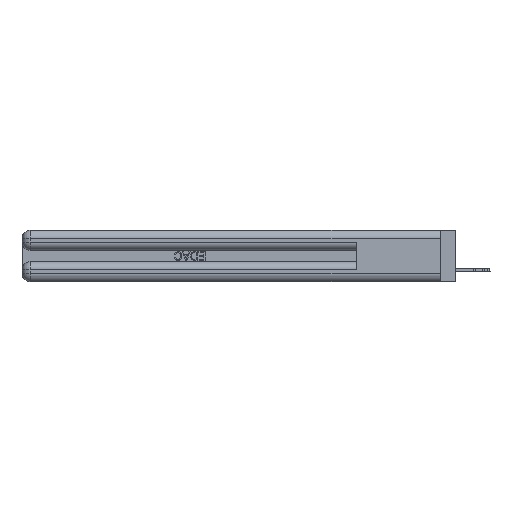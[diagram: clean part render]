
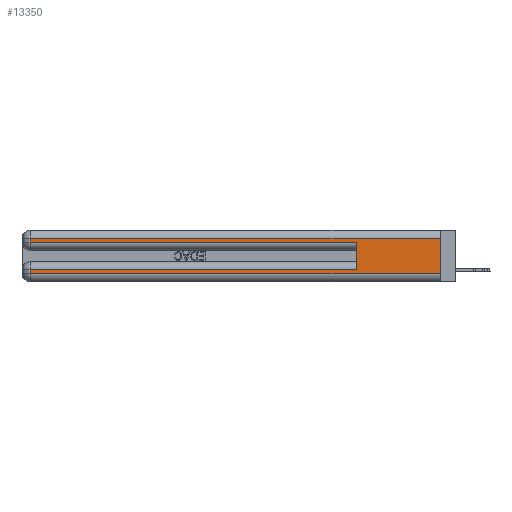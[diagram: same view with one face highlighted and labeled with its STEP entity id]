
A CAD part, left-side view. The second image highlights one B-rep face of the part: STEP entity #13350.
In plain terms, the highlighted planar face has unit normal (-1, 0, 0).
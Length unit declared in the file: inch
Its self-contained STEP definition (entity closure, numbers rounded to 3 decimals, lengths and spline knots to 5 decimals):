
#110 = DIRECTION ( 'NONE',  ( 0., 0., -1. ) ) ;
#806 = VERTEX_POINT ( 'NONE', #2833 ) ;
#1689 = VECTOR ( 'NONE', #25613, 39.37008 ) ;
#2033 = EDGE_CURVE ( 'NONE', #21175, #6465, #29939, .T. ) ;
#2107 = EDGE_CURVE ( 'NONE', #31301, #806, #5621, .T. ) ;
#2484 = FACE_OUTER_BOUND ( 'NONE', #23360, .T. ) ;
#2603 = DIRECTION ( 'NONE',  ( 0., 0., -1. ) ) ;
#2833 = CARTESIAN_POINT ( 'NONE',  ( 0., 2.94, 0.285 ) ) ;
#2837 = ORIENTED_EDGE ( 'NONE', *, *, #35792, .T. ) ;
#3821 = CARTESIAN_POINT ( 'NONE',  ( 0., 0., 0.085 ) ) ;
#3968 = DIRECTION ( 'NONE',  ( 0., 1., 0. ) ) ;
#4690 = ORIENTED_EDGE ( 'NONE', *, *, #9439, .F. ) ;
#5583 = AXIS2_PLACEMENT_3D ( 'NONE', #5845, #15861, #2603 ) ;
#5621 = LINE ( 'NONE', #41473, #11969 ) ;
#5845 = CARTESIAN_POINT ( 'NONE',  ( 0., 0., 0.37 ) ) ;
#6465 = VERTEX_POINT ( 'NONE', #33110 ) ;
#7440 = LINE ( 'NONE', #3821, #31172 ) ;
#9402 = CARTESIAN_POINT ( 'NONE',  ( 0., 2.94, 0.085 ) ) ;
#9439 = EDGE_CURVE ( 'NONE', #25438, #43082, #18098, .T. ) ;
#9541 = PLANE ( 'NONE',  #5583 ) ;
#10227 = VECTOR ( 'NONE', #19446, 39.37008 ) ;
#10429 = CARTESIAN_POINT ( 'NONE',  ( 0., 2.94, 0.31 ) ) ;
#11605 = CARTESIAN_POINT ( 'NONE',  ( 0., 2.94, 0.06 ) ) ;
#11969 = VECTOR ( 'NONE', #35269, 39.37008 ) ;
#12054 = CARTESIAN_POINT ( 'NONE',  ( 0., 0., 0.31 ) ) ;
#13350 = ADVANCED_FACE ( 'NONE', ( #2484 ), #9541, .F. ) ;
#14698 = EDGE_CURVE ( 'NONE', #25438, #38427, #7440, .T. ) ;
#15668 = CARTESIAN_POINT ( 'NONE',  ( 0., 0., 0.285 ) ) ;
#15861 = DIRECTION ( 'NONE',  ( 1., 0., 0. ) ) ;
#16443 = LINE ( 'NONE', #21924, #1689 ) ;
#16567 = CARTESIAN_POINT ( 'NONE',  ( 0., 0., 0.37 ) ) ;
#16701 = VECTOR ( 'NONE', #39273, 39.37008 ) ;
#17073 = EDGE_CURVE ( 'NONE', #38427, #19320, #24148, .T. ) ;
#17250 = CARTESIAN_POINT ( 'NONE',  ( 0., 0.6, 0.085 ) ) ;
#17826 = ORIENTED_EDGE ( 'NONE', *, *, #21265, .T. ) ;
#18098 = LINE ( 'NONE', #42594, #10227 ) ;
#19320 = VERTEX_POINT ( 'NONE', #11605 ) ;
#19446 = DIRECTION ( 'NONE',  ( 0., 0., 1. ) ) ;
#20258 = ORIENTED_EDGE ( 'NONE', *, *, #2107, .T. ) ;
#20483 = ORIENTED_EDGE ( 'NONE', *, *, #38315, .T. ) ;
#21175 = VERTEX_POINT ( 'NONE', #12054 ) ;
#21265 = EDGE_CURVE ( 'NONE', #21175, #31301, #34401, .T. ) ;
#21924 = CARTESIAN_POINT ( 'NONE',  ( 0., 0., 0.06 ) ) ;
#23090 = DIRECTION ( 'NONE',  ( 0., 1., 0. ) ) ;
#23360 = EDGE_LOOP ( 'NONE', ( #40147, #17826, #20258, #2837, #4690, #25786, #35320, #20483 ) ) ;
#24148 = LINE ( 'NONE', #43578, #26282 ) ;
#25367 = CARTESIAN_POINT ( 'NONE',  ( 0., 0.6, 0.285 ) ) ;
#25438 = VERTEX_POINT ( 'NONE', #17250 ) ;
#25613 = DIRECTION ( 'NONE',  ( 0., -1., 0. ) ) ;
#25664 = LINE ( 'NONE', #15668, #16701 ) ;
#25786 = ORIENTED_EDGE ( 'NONE', *, *, #14698, .T. ) ;
#26282 = VECTOR ( 'NONE', #110, 39.37008 ) ;
#29939 = LINE ( 'NONE', #16567, #31486 ) ;
#31172 = VECTOR ( 'NONE', #3968, 39.37008 ) ;
#31301 = VERTEX_POINT ( 'NONE', #10429 ) ;
#31486 = VECTOR ( 'NONE', #43559, 39.37008 ) ;
#33110 = CARTESIAN_POINT ( 'NONE',  ( 0., 0., 0.06 ) ) ;
#33892 = VECTOR ( 'NONE', #23090, 39.37008 ) ;
#34401 = LINE ( 'NONE', #43290, #33892 ) ;
#35269 = DIRECTION ( 'NONE',  ( 0., 0., -1. ) ) ;
#35320 = ORIENTED_EDGE ( 'NONE', *, *, #17073, .T. ) ;
#35792 = EDGE_CURVE ( 'NONE', #806, #43082, #25664, .T. ) ;
#38315 = EDGE_CURVE ( 'NONE', #19320, #6465, #16443, .T. ) ;
#38427 = VERTEX_POINT ( 'NONE', #9402 ) ;
#39273 = DIRECTION ( 'NONE',  ( 0., -1., 0. ) ) ;
#40147 = ORIENTED_EDGE ( 'NONE', *, *, #2033, .F. ) ;
#41473 = CARTESIAN_POINT ( 'NONE',  ( 0., 2.94, 0.37 ) ) ;
#42594 = CARTESIAN_POINT ( 'NONE',  ( 0., 0.6, 0.145 ) ) ;
#43082 = VERTEX_POINT ( 'NONE', #25367 ) ;
#43290 = CARTESIAN_POINT ( 'NONE',  ( 0., 0., 0.31 ) ) ;
#43559 = DIRECTION ( 'NONE',  ( 0., 0., -1. ) ) ;
#43578 = CARTESIAN_POINT ( 'NONE',  ( 0., 2.94, 0.37 ) ) ;
